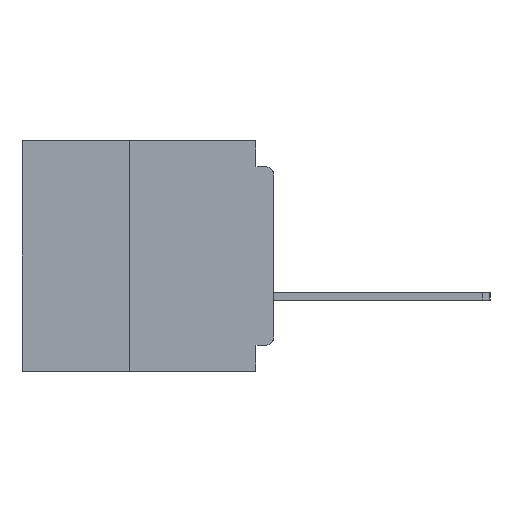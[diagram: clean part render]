
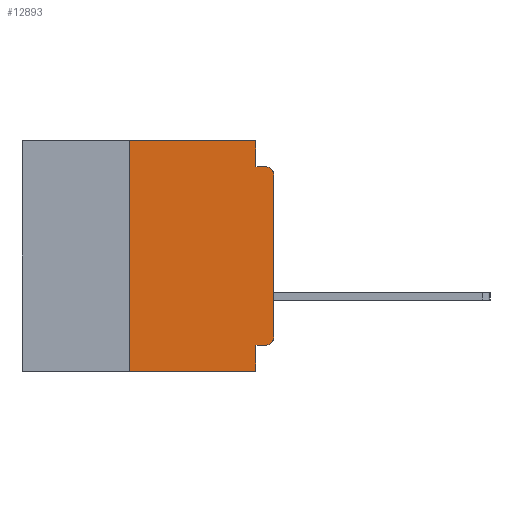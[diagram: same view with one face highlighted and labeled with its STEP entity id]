
A CAD part, left-side view. The second image highlights one B-rep face of the part: STEP entity #12893.
In plain terms, the highlighted planar face has unit normal (-1, 0, 0).
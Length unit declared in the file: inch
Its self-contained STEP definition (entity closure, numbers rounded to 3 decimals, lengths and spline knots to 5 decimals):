
#381 = ORIENTED_EDGE ( 'NONE', *, *, #4654, .T. ) ;
#744 = CARTESIAN_POINT ( 'NONE',  ( 0., 0.015, -0.355 ) ) ;
#949 = CARTESIAN_POINT ( 'NONE',  ( 0., 0.437, 0. ) ) ;
#1117 = CARTESIAN_POINT ( 'NONE',  ( 0., 0.25, -0.4 ) ) ;
#1244 = DIRECTION ( 'NONE',  ( 1., 0., 0. ) ) ;
#2142 = CARTESIAN_POINT ( 'NONE',  ( 0., 0.25, 0. ) ) ;
#2816 = VERTEX_POINT ( 'NONE', #39858 ) ;
#3123 = CARTESIAN_POINT ( 'NONE',  ( 0., 0., -0.355 ) ) ;
#3180 = CIRCLE ( 'NONE', #9103, 0.015 ) ;
#3649 = VECTOR ( 'NONE', #28965, 39.37008 ) ;
#3685 = LINE ( 'NONE', #19357, #25646 ) ;
#4625 = VERTEX_POINT ( 'NONE', #10287 ) ;
#4654 = EDGE_CURVE ( 'NONE', #17601, #4625, #3180, .T. ) ;
#5428 = AXIS2_PLACEMENT_3D ( 'NONE', #7397, #40059, #12073 ) ;
#5525 = DIRECTION ( 'NONE',  ( 0., -1., 0. ) ) ;
#5563 = CARTESIAN_POINT ( 'NONE',  ( 0., 0.031, -0.4 ) ) ;
#5867 = DIRECTION ( 'NONE',  ( 0., 0., 1. ) ) ;
#6424 = VERTEX_POINT ( 'NONE', #43138 ) ;
#6632 = EDGE_CURVE ( 'NONE', #28054, #17049, #59017, .T. ) ;
#7397 = CARTESIAN_POINT ( 'NONE',  ( 0., 0.015, -0.34 ) ) ;
#9103 = AXIS2_PLACEMENT_3D ( 'NONE', #19850, #52360, #24582 ) ;
#9182 = VECTOR ( 'NONE', #45381, 39.37008 ) ;
#9335 = VERTEX_POINT ( 'NONE', #38769 ) ;
#10287 = CARTESIAN_POINT ( 'NONE',  ( 0., 0.015, -0.045 ) ) ;
#10631 = LINE ( 'NONE', #49611, #9182 ) ;
#10864 = EDGE_CURVE ( 'NONE', #6424, #17601, #52382, .T. ) ;
#11047 = VECTOR ( 'NONE', #35808, 39.37008 ) ;
#11612 = ORIENTED_EDGE ( 'NONE', *, *, #37280, .F. ) ;
#12073 = DIRECTION ( 'NONE',  ( 0., 0., -1. ) ) ;
#12236 = EDGE_CURVE ( 'NONE', #9335, #34342, #57267, .T. ) ;
#12893 = ADVANCED_FACE ( 'NONE', ( #37081 ), #24565, .F. ) ;
#13508 = ORIENTED_EDGE ( 'NONE', *, *, #12236, .F. ) ;
#14327 = ORIENTED_EDGE ( 'NONE', *, *, #38274, .T. ) ;
#15303 = VECTOR ( 'NONE', #60046, 39.37008 ) ;
#16073 = LINE ( 'NONE', #949, #3649 ) ;
#16346 = ORIENTED_EDGE ( 'NONE', *, *, #38254, .F. ) ;
#17049 = VERTEX_POINT ( 'NONE', #58459 ) ;
#17601 = VERTEX_POINT ( 'NONE', #29827 ) ;
#18943 = ORIENTED_EDGE ( 'NONE', *, *, #56921, .F. ) ;
#19357 = CARTESIAN_POINT ( 'NONE',  ( 0., 0.437, -0.4 ) ) ;
#19614 = EDGE_CURVE ( 'NONE', #17049, #2816, #41937, .T. ) ;
#19850 = CARTESIAN_POINT ( 'NONE',  ( 0., 0.015, -0.06 ) ) ;
#24565 = PLANE ( 'NONE',  #42239 ) ;
#24582 = DIRECTION ( 'NONE',  ( 0., 0., -1. ) ) ;
#25646 = VECTOR ( 'NONE', #5525, 39.37008 ) ;
#25928 = EDGE_CURVE ( 'NONE', #9335, #2816, #3685, .T. ) ;
#26625 = VECTOR ( 'NONE', #42875, 39.37008 ) ;
#28054 = VERTEX_POINT ( 'NONE', #744 ) ;
#28965 = DIRECTION ( 'NONE',  ( 0., -1., 0. ) ) ;
#29410 = EDGE_LOOP ( 'NONE', ( #48557, #381, #16346, #11612, #18943, #13508, #56373, #47219, #52255, #14327 ) ) ;
#29827 = CARTESIAN_POINT ( 'NONE',  ( 0., 0., -0.06 ) ) ;
#30449 = DIRECTION ( 'NONE',  ( 0., -1., 0. ) ) ;
#30766 = VERTEX_POINT ( 'NONE', #48857 ) ;
#32664 = VECTOR ( 'NONE', #5867, 39.37008 ) ;
#33963 = DIRECTION ( 'NONE',  ( 0., 0., -1. ) ) ;
#34342 = VERTEX_POINT ( 'NONE', #2142 ) ;
#35808 = DIRECTION ( 'NONE',  ( 0., 1., 0. ) ) ;
#37081 = FACE_OUTER_BOUND ( 'NONE', #29410, .T. ) ;
#37280 = EDGE_CURVE ( 'NONE', #30766, #43154, #10631, .T. ) ;
#37904 = CIRCLE ( 'NONE', #5428, 0.015 ) ;
#38254 = EDGE_CURVE ( 'NONE', #43154, #4625, #51597, .T. ) ;
#38274 = EDGE_CURVE ( 'NONE', #28054, #6424, #37904, .T. ) ;
#38769 = CARTESIAN_POINT ( 'NONE',  ( 0., 0.25, -0.4 ) ) ;
#39354 = VECTOR ( 'NONE', #30449, 39.37008 ) ;
#39858 = CARTESIAN_POINT ( 'NONE',  ( 0., 0.031, -0.4 ) ) ;
#40059 = DIRECTION ( 'NONE',  ( -1., 0., 0. ) ) ;
#41937 = LINE ( 'NONE', #5563, #26625 ) ;
#42239 = AXIS2_PLACEMENT_3D ( 'NONE', #57002, #1244, #33963 ) ;
#42875 = DIRECTION ( 'NONE',  ( 0., 0., -1. ) ) ;
#43138 = CARTESIAN_POINT ( 'NONE',  ( 0., 0., -0.34 ) ) ;
#43154 = VERTEX_POINT ( 'NONE', #58240 ) ;
#45381 = DIRECTION ( 'NONE',  ( 0., 0., -1. ) ) ;
#47219 = ORIENTED_EDGE ( 'NONE', *, *, #19614, .F. ) ;
#48557 = ORIENTED_EDGE ( 'NONE', *, *, #10864, .T. ) ;
#48857 = CARTESIAN_POINT ( 'NONE',  ( 0., 0.031, 0. ) ) ;
#49611 = CARTESIAN_POINT ( 'NONE',  ( 0., 0.031, 0. ) ) ;
#51597 = LINE ( 'NONE', #58188, #39354 ) ;
#52255 = ORIENTED_EDGE ( 'NONE', *, *, #6632, .F. ) ;
#52360 = DIRECTION ( 'NONE',  ( -1., 0., 0. ) ) ;
#52382 = LINE ( 'NONE', #55418, #15303 ) ;
#55418 = CARTESIAN_POINT ( 'NONE',  ( 0., 0., 0. ) ) ;
#56373 = ORIENTED_EDGE ( 'NONE', *, *, #25928, .T. ) ;
#56921 = EDGE_CURVE ( 'NONE', #34342, #30766, #16073, .T. ) ;
#57002 = CARTESIAN_POINT ( 'NONE',  ( 0., 0.437, 0. ) ) ;
#57267 = LINE ( 'NONE', #1117, #32664 ) ;
#58188 = CARTESIAN_POINT ( 'NONE',  ( 0., 0., -0.045 ) ) ;
#58240 = CARTESIAN_POINT ( 'NONE',  ( 0., 0.031, -0.045 ) ) ;
#58459 = CARTESIAN_POINT ( 'NONE',  ( 0., 0.031, -0.355 ) ) ;
#59017 = LINE ( 'NONE', #3123, #11047 ) ;
#60046 = DIRECTION ( 'NONE',  ( 0., 0., 1. ) ) ;
